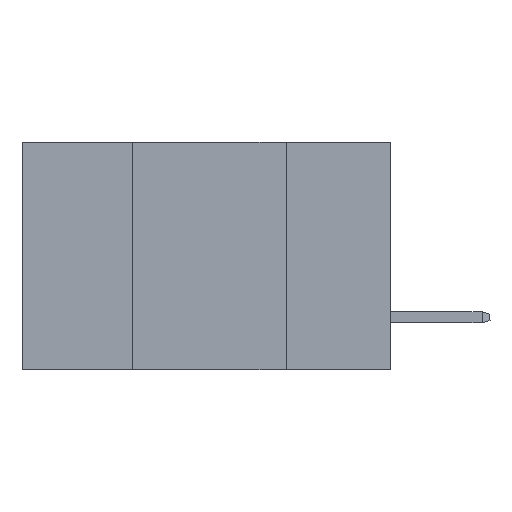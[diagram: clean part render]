
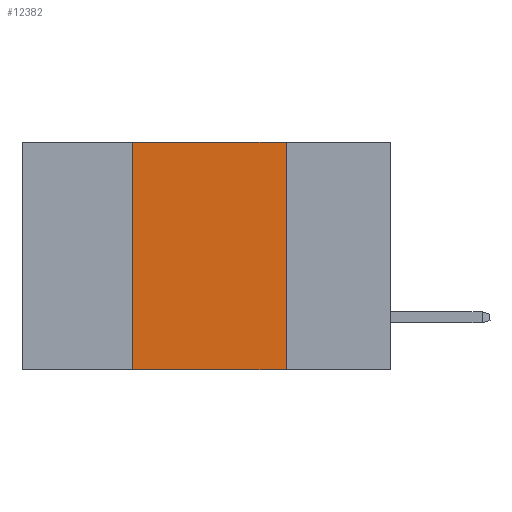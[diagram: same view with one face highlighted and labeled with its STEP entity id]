
A CAD part, left-side view. The second image highlights one B-rep face of the part: STEP entity #12382.
In plain terms, the highlighted planar face has unit normal (-1, 0, 0).
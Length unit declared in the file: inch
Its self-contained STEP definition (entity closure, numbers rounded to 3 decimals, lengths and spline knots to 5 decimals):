
#385 = LINE ( 'NONE', #899, #6363 ) ;
#848 = DIRECTION ( 'NONE',  ( 0., -1., 0. ) ) ;
#899 = CARTESIAN_POINT ( 'NONE',  ( 0., 0.6, -0.37 ) ) ;
#920 = VERTEX_POINT ( 'NONE', #6844 ) ;
#1112 = EDGE_LOOP ( 'NONE', ( #4775, #4877, #10270, #6444 ) ) ;
#3603 = EDGE_CURVE ( 'NONE', #5453, #920, #5376, .T. ) ;
#3829 = EDGE_CURVE ( 'NONE', #5809, #6708, #9550, .T. ) ;
#3881 = LINE ( 'NONE', #13696, #6451 ) ;
#4203 = EDGE_CURVE ( 'NONE', #5809, #920, #385, .T. ) ;
#4451 = PLANE ( 'NONE',  #10720 ) ;
#4775 = ORIENTED_EDGE ( 'NONE', *, *, #3603, .F. ) ;
#4877 = ORIENTED_EDGE ( 'NONE', *, *, #10149, .F. ) ;
#5376 = LINE ( 'NONE', #11241, #5532 ) ;
#5453 = VERTEX_POINT ( 'NONE', #8629 ) ;
#5532 = VECTOR ( 'NONE', #12282, 39.37008 ) ;
#5605 = DIRECTION ( 'NONE',  ( 1., 0., 0. ) ) ;
#5809 = VERTEX_POINT ( 'NONE', #8241 ) ;
#6075 = FACE_OUTER_BOUND ( 'NONE', #1112, .T. ) ;
#6363 = VECTOR ( 'NONE', #848, 39.37008 ) ;
#6444 = ORIENTED_EDGE ( 'NONE', *, *, #4203, .T. ) ;
#6451 = VECTOR ( 'NONE', #6831, 39.37008 ) ;
#6694 = VECTOR ( 'NONE', #7117, 39.37008 ) ;
#6708 = VERTEX_POINT ( 'NONE', #12963 ) ;
#6831 = DIRECTION ( 'NONE',  ( 0., -1., 0. ) ) ;
#6844 = CARTESIAN_POINT ( 'NONE',  ( 0., 0.17, -0.37 ) ) ;
#7117 = DIRECTION ( 'NONE',  ( 0., 0., 1. ) ) ;
#7132 = CARTESIAN_POINT ( 'NONE',  ( 0., 0.42, 0. ) ) ;
#8241 = CARTESIAN_POINT ( 'NONE',  ( 0., 0.42, -0.37 ) ) ;
#8629 = CARTESIAN_POINT ( 'NONE',  ( 0., 0.17, 0. ) ) ;
#9550 = LINE ( 'NONE', #7132, #6694 ) ;
#10149 = EDGE_CURVE ( 'NONE', #6708, #5453, #3881, .T. ) ;
#10270 = ORIENTED_EDGE ( 'NONE', *, *, #3829, .F. ) ;
#10720 = AXIS2_PLACEMENT_3D ( 'NONE', #11516, #5605, #12547 ) ;
#11241 = CARTESIAN_POINT ( 'NONE',  ( 0., 0.17, 0. ) ) ;
#11516 = CARTESIAN_POINT ( 'NONE',  ( 0., 0.6, 0. ) ) ;
#12282 = DIRECTION ( 'NONE',  ( 0., 0., -1. ) ) ;
#12382 = ADVANCED_FACE ( 'NONE', ( #6075 ), #4451, .F. ) ;
#12547 = DIRECTION ( 'NONE',  ( 0., 0., -1. ) ) ;
#12963 = CARTESIAN_POINT ( 'NONE',  ( 0., 0.42, 0. ) ) ;
#13696 = CARTESIAN_POINT ( 'NONE',  ( 0., 0.6, 0. ) ) ;
